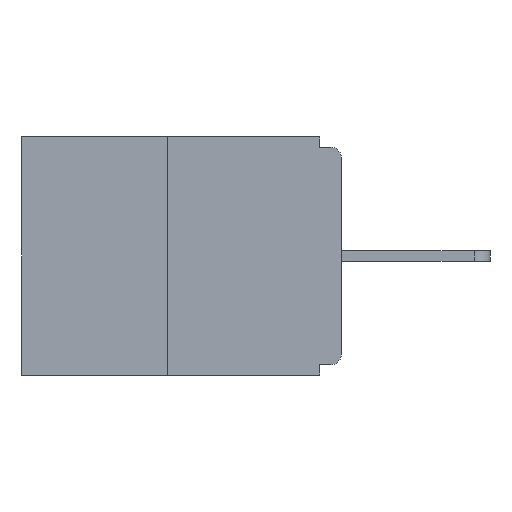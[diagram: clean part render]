
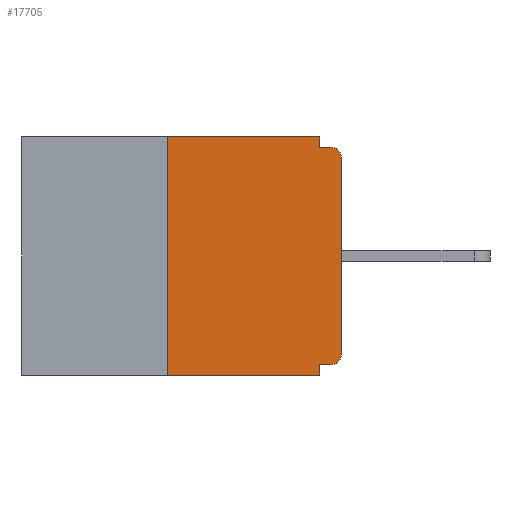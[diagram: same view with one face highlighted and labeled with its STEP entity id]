
A CAD part, left-side view. The second image highlights one B-rep face of the part: STEP entity #17705.
In plain terms, the highlighted planar face has unit normal (-1, 0, 0).
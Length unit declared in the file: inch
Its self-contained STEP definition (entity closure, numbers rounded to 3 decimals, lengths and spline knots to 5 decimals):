
#223 = CARTESIAN_POINT ( 'NONE',  ( 0., 0.031, 0. ) ) ;
#434 = LINE ( 'NONE', #15826, #3969 ) ;
#537 = AXIS2_PLACEMENT_3D ( 'NONE', #6352, #16892, #7846 ) ;
#886 = CARTESIAN_POINT ( 'NONE',  ( 0., 0.015, -0.015 ) ) ;
#1149 = EDGE_CURVE ( 'NONE', #8208, #10975, #18031, .T. ) ;
#1400 = EDGE_CURVE ( 'NONE', #17148, #18147, #9364, .T. ) ;
#1537 = VECTOR ( 'NONE', #8973, 39.37008 ) ;
#1678 = CARTESIAN_POINT ( 'NONE',  ( 0., 0.031, -0.015 ) ) ;
#2029 = CARTESIAN_POINT ( 'NONE',  ( 0., 0., -0.03 ) ) ;
#2088 = VERTEX_POINT ( 'NONE', #18732 ) ;
#2377 = VERTEX_POINT ( 'NONE', #16347 ) ;
#3280 = EDGE_CURVE ( 'NONE', #2377, #19333, #11794, .T. ) ;
#3684 = CARTESIAN_POINT ( 'NONE',  ( 0., 0.015, -0.03 ) ) ;
#3757 = VECTOR ( 'NONE', #9310, 39.37008 ) ;
#3948 = DIRECTION ( 'NONE',  ( 1., 0., 0. ) ) ;
#3969 = VECTOR ( 'NONE', #14270, 39.37008 ) ;
#3983 = VECTOR ( 'NONE', #10384, 39.37008 ) ;
#4010 = ORIENTED_EDGE ( 'NONE', *, *, #7207, .F. ) ;
#4021 = ORIENTED_EDGE ( 'NONE', *, *, #1149, .F. ) ;
#4027 = ORIENTED_EDGE ( 'NONE', *, *, #12619, .T. ) ;
#4055 = EDGE_LOOP ( 'NONE', ( #4010, #4021, #4027, #4124, #4177, #4280, #4373, #4416, #4478, #4541 ) ) ;
#4124 = ORIENTED_EDGE ( 'NONE', *, *, #18766, .F. ) ;
#4144 = VERTEX_POINT ( 'NONE', #1678 ) ;
#4177 = ORIENTED_EDGE ( 'NONE', *, *, #3280, .F. ) ;
#4280 = ORIENTED_EDGE ( 'NONE', *, *, #9504, .T. ) ;
#4373 = ORIENTED_EDGE ( 'NONE', *, *, #1400, .T. ) ;
#4416 = ORIENTED_EDGE ( 'NONE', *, *, #7815, .T. ) ;
#4458 = LINE ( 'NONE', #8884, #3983 ) ;
#4478 = ORIENTED_EDGE ( 'NONE', *, *, #9113, .F. ) ;
#4529 = DIRECTION ( 'NONE',  ( 0., -1., 0. ) ) ;
#4541 = ORIENTED_EDGE ( 'NONE', *, *, #12726, .F. ) ;
#5219 = DIRECTION ( 'NONE',  ( 0., 0., -1. ) ) ;
#5664 = VECTOR ( 'NONE', #4529, 39.37008 ) ;
#6311 = LINE ( 'NONE', #6967, #18282 ) ;
#6352 = CARTESIAN_POINT ( 'NONE',  ( 0., 0.015, -0.313 ) ) ;
#6793 = AXIS2_PLACEMENT_3D ( 'NONE', #11379, #3948, #14510 ) ;
#6967 = CARTESIAN_POINT ( 'NONE',  ( 0., 0., -0.015 ) ) ;
#7207 = EDGE_CURVE ( 'NONE', #10975, #8126, #434, .T. ) ;
#7690 = CARTESIAN_POINT ( 'NONE',  ( 0., 0.25, -0.343 ) ) ;
#7815 = EDGE_CURVE ( 'NONE', #18147, #16612, #8485, .T. ) ;
#7846 = DIRECTION ( 'NONE',  ( 0., 0., -1. ) ) ;
#8126 = VERTEX_POINT ( 'NONE', #10608 ) ;
#8208 = VERTEX_POINT ( 'NONE', #7690 ) ;
#8485 = CIRCLE ( 'NONE', #18291, 0.015 ) ;
#8771 = FACE_OUTER_BOUND ( 'NONE', #4055, .T. ) ;
#8884 = CARTESIAN_POINT ( 'NONE',  ( 0., 0.031, -0.343 ) ) ;
#8973 = DIRECTION ( 'NONE',  ( 0., 0., 1. ) ) ;
#9113 = EDGE_CURVE ( 'NONE', #4144, #16612, #6311, .T. ) ;
#9227 = LINE ( 'NONE', #13547, #5664 ) ;
#9310 = DIRECTION ( 'NONE',  ( 0., 0., -1. ) ) ;
#9364 = LINE ( 'NONE', #18127, #12817 ) ;
#9504 = EDGE_CURVE ( 'NONE', #2377, #17148, #11662, .T. ) ;
#10384 = DIRECTION ( 'NONE',  ( 0., 0., -1. ) ) ;
#10608 = CARTESIAN_POINT ( 'NONE',  ( 0., 0.031, 0. ) ) ;
#10893 = VECTOR ( 'NONE', #15007, 39.37008 ) ;
#10975 = VERTEX_POINT ( 'NONE', #13717 ) ;
#11379 = CARTESIAN_POINT ( 'NONE',  ( 0., 0.46, 0. ) ) ;
#11553 = CARTESIAN_POINT ( 'NONE',  ( 0., 0.25, 0. ) ) ;
#11662 = CIRCLE ( 'NONE', #537, 0.015 ) ;
#11744 = LINE ( 'NONE', #223, #3757 ) ;
#11794 = LINE ( 'NONE', #15035, #10893 ) ;
#12619 = EDGE_CURVE ( 'NONE', #8208, #2088, #9227, .T. ) ;
#12726 = EDGE_CURVE ( 'NONE', #8126, #4144, #11744, .T. ) ;
#12817 = VECTOR ( 'NONE', #18261, 39.37008 ) ;
#12949 = PLANE ( 'NONE',  #6793 ) ;
#13291 = CARTESIAN_POINT ( 'NONE',  ( 0., 0.031, -0.328 ) ) ;
#13547 = CARTESIAN_POINT ( 'NONE',  ( 0., 0.46, -0.343 ) ) ;
#13717 = CARTESIAN_POINT ( 'NONE',  ( 0., 0.25, 0. ) ) ;
#14249 = DIRECTION ( 'NONE',  ( -1., 0., 0. ) ) ;
#14270 = DIRECTION ( 'NONE',  ( 0., -1., 0. ) ) ;
#14278 = CARTESIAN_POINT ( 'NONE',  ( 0., 0., -0.313 ) ) ;
#14510 = DIRECTION ( 'NONE',  ( 0., 0., -1. ) ) ;
#15007 = DIRECTION ( 'NONE',  ( 0., 1., 0. ) ) ;
#15035 = CARTESIAN_POINT ( 'NONE',  ( 0., 0., -0.328 ) ) ;
#15826 = CARTESIAN_POINT ( 'NONE',  ( 0., 0.46, 0. ) ) ;
#16347 = CARTESIAN_POINT ( 'NONE',  ( 0., 0.015, -0.328 ) ) ;
#16612 = VERTEX_POINT ( 'NONE', #886 ) ;
#16892 = DIRECTION ( 'NONE',  ( -1., 0., 0. ) ) ;
#17148 = VERTEX_POINT ( 'NONE', #14278 ) ;
#17485 = DIRECTION ( 'NONE',  ( 0., -1., 0. ) ) ;
#17705 = ADVANCED_FACE ( 'NONE', ( #8771 ), #12949, .F. ) ;
#18031 = LINE ( 'NONE', #11553, #1537 ) ;
#18127 = CARTESIAN_POINT ( 'NONE',  ( 0., 0., 0. ) ) ;
#18147 = VERTEX_POINT ( 'NONE', #2029 ) ;
#18261 = DIRECTION ( 'NONE',  ( 0., 0., 1. ) ) ;
#18282 = VECTOR ( 'NONE', #17485, 39.37008 ) ;
#18291 = AXIS2_PLACEMENT_3D ( 'NONE', #3684, #14249, #5219 ) ;
#18732 = CARTESIAN_POINT ( 'NONE',  ( 0., 0.031, -0.343 ) ) ;
#18766 = EDGE_CURVE ( 'NONE', #19333, #2088, #4458, .T. ) ;
#19333 = VERTEX_POINT ( 'NONE', #13291 ) ;
